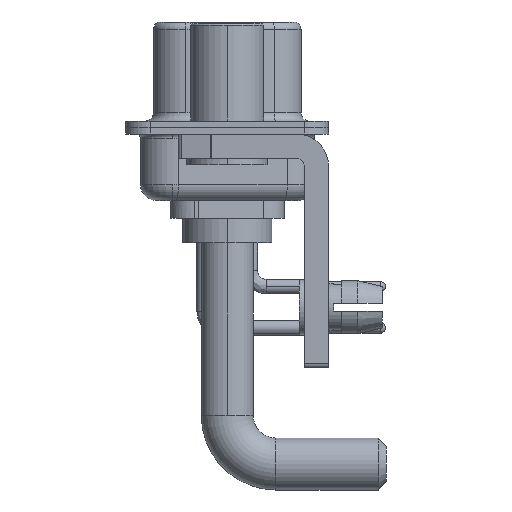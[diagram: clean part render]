
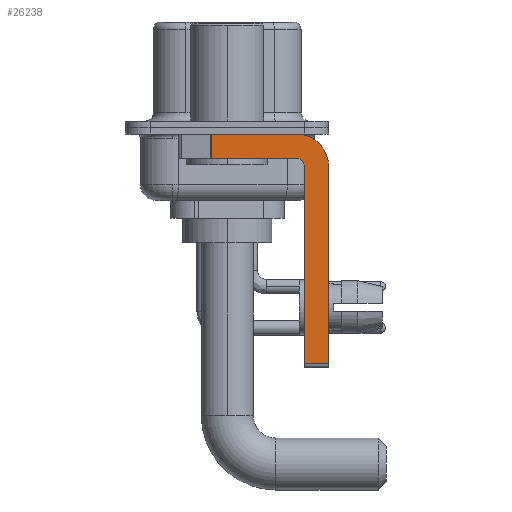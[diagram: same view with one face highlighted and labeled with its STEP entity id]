
A CAD part, left-side view. The second image highlights one B-rep face of the part: STEP entity #26238.
In plain terms, the highlighted planar face has unit normal (-1, 0, 0).
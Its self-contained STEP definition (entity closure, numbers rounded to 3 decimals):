
#71 = ORIENTED_EDGE ( 'NONE', *, *, #15314, .F. ) ;
#150 = CARTESIAN_POINT ( 'NONE',  ( -2.9, -4.25, -2.4 ) ) ;
#545 = CARTESIAN_POINT ( 'NONE',  ( -2.9, -4.25, -14.55 ) ) ;
#1232 = DIRECTION ( 'NONE',  ( -1., 0., 0. ) ) ;
#1467 = ORIENTED_EDGE ( 'NONE', *, *, #22378, .F. ) ;
#1584 = CARTESIAN_POINT ( 'NONE',  ( -2.9, -4.75, -2.4 ) ) ;
#1608 = VECTOR ( 'NONE', #7504, 1000. ) ;
#1879 = DIRECTION ( 'NONE',  ( 1., 0., 0. ) ) ;
#2025 = DIRECTION ( 'NONE',  ( 0., 0., -1. ) ) ;
#2563 = ORIENTED_EDGE ( 'NONE', *, *, #26449, .T. ) ;
#2705 = EDGE_LOOP ( 'NONE', ( #11683, #2563, #71, #1467, #7430, #20821, #26855, #7572 ) ) ;
#4264 = VECTOR ( 'NONE', #14315, 1000. ) ;
#5540 = CARTESIAN_POINT ( 'NONE',  ( -2.9, -6.25, -2.4 ) ) ;
#6569 = DIRECTION ( 'NONE',  ( 0., -1., 0. ) ) ;
#6678 = CIRCLE ( 'NONE', #23451, 2. ) ;
#7073 = LINE ( 'NONE', #20624, #1608 ) ;
#7117 = DIRECTION ( 'NONE',  ( 0., -1., 0. ) ) ;
#7430 = ORIENTED_EDGE ( 'NONE', *, *, #21015, .F. ) ;
#7504 = DIRECTION ( 'NONE',  ( 0., 0., 1. ) ) ;
#7505 = EDGE_CURVE ( 'NONE', #22199, #14180, #24375, .T. ) ;
#7572 = ORIENTED_EDGE ( 'NONE', *, *, #18465, .F. ) ;
#7615 = AXIS2_PLACEMENT_3D ( 'NONE', #12761, #1232, #8510 ) ;
#8292 = VERTEX_POINT ( 'NONE', #28421 ) ;
#8510 = DIRECTION ( 'NONE',  ( 0., 0., 1. ) ) ;
#8869 = CARTESIAN_POINT ( 'NONE',  ( -2.9, 0.978, -1.9 ) ) ;
#9920 = LINE ( 'NONE', #5540, #4264 ) ;
#10134 = VERTEX_POINT ( 'NONE', #26465 ) ;
#11087 = CARTESIAN_POINT ( 'NONE',  ( -2.9, 3., -0.4 ) ) ;
#11683 = ORIENTED_EDGE ( 'NONE', *, *, #7505, .F. ) ;
#12678 = CARTESIAN_POINT ( 'NONE',  ( -2.9, 0.978, -1.9 ) ) ;
#12738 = CARTESIAN_POINT ( 'NONE',  ( -2.9, -4.25, -1.9 ) ) ;
#12761 = CARTESIAN_POINT ( 'NONE',  ( -2.9, -4.25, -2.4 ) ) ;
#12811 = VERTEX_POINT ( 'NONE', #12738 ) ;
#13073 = EDGE_CURVE ( 'NONE', #8292, #20389, #9920, .T. ) ;
#13638 = VERTEX_POINT ( 'NONE', #1584 ) ;
#13811 = VECTOR ( 'NONE', #7117, 1000. ) ;
#14180 = VERTEX_POINT ( 'NONE', #19764 ) ;
#14315 = DIRECTION ( 'NONE',  ( 0., 0., -1. ) ) ;
#14385 = LINE ( 'NONE', #18903, #27163 ) ;
#15314 = EDGE_CURVE ( 'NONE', #12811, #18413, #14385, .T. ) ;
#15554 = CARTESIAN_POINT ( 'NONE',  ( -2.9, 0.978, -0.4 ) ) ;
#15763 = FACE_OUTER_BOUND ( 'NONE', #2705, .T. ) ;
#16015 = CARTESIAN_POINT ( 'NONE',  ( -2.9, -6.25, -14.55 ) ) ;
#18363 = CARTESIAN_POINT ( 'NONE',  ( -2.9, -4.25, -2.4 ) ) ;
#18413 = VERTEX_POINT ( 'NONE', #8869 ) ;
#18465 = EDGE_CURVE ( 'NONE', #14180, #8292, #6678, .T. ) ;
#18903 = CARTESIAN_POINT ( 'NONE',  ( -2.9, -4.25, -1.9 ) ) ;
#19764 = CARTESIAN_POINT ( 'NONE',  ( -2.9, -4.25, -0.4 ) ) ;
#19824 = VECTOR ( 'NONE', #2025, 1000. ) ;
#20389 = VERTEX_POINT ( 'NONE', #16015 ) ;
#20624 = CARTESIAN_POINT ( 'NONE',  ( -2.9, -4.75, -14.8 ) ) ;
#20754 = AXIS2_PLACEMENT_3D ( 'NONE', #150, #1879, #22744 ) ;
#20795 = DIRECTION ( 'NONE',  ( 0., 1., 0. ) ) ;
#20821 = ORIENTED_EDGE ( 'NONE', *, *, #26730, .T. ) ;
#20839 = LINE ( 'NONE', #12678, #19824 ) ;
#21015 = EDGE_CURVE ( 'NONE', #10134, #13638, #7073, .T. ) ;
#22199 = VERTEX_POINT ( 'NONE', #15554 ) ;
#22378 = EDGE_CURVE ( 'NONE', #13638, #12811, #24372, .T. ) ;
#22744 = DIRECTION ( 'NONE',  ( 0., 0., -1. ) ) ;
#23451 = AXIS2_PLACEMENT_3D ( 'NONE', #18363, #25754, #27278 ) ;
#24372 = CIRCLE ( 'NONE', #7615, 0.5 ) ;
#24375 = LINE ( 'NONE', #11087, #26717 ) ;
#25754 = DIRECTION ( 'NONE',  ( 1., 0., 0. ) ) ;
#26238 = ADVANCED_FACE ( 'NONE', ( #15763 ), #27306, .F. ) ;
#26449 = EDGE_CURVE ( 'NONE', #22199, #18413, #20839, .T. ) ;
#26465 = CARTESIAN_POINT ( 'NONE',  ( -2.9, -4.75, -14.55 ) ) ;
#26717 = VECTOR ( 'NONE', #6569, 1000. ) ;
#26730 = EDGE_CURVE ( 'NONE', #10134, #20389, #27111, .T. ) ;
#26855 = ORIENTED_EDGE ( 'NONE', *, *, #13073, .F. ) ;
#27111 = LINE ( 'NONE', #545, #13811 ) ;
#27163 = VECTOR ( 'NONE', #20795, 1000. ) ;
#27278 = DIRECTION ( 'NONE',  ( 0., 0., -1. ) ) ;
#27306 = PLANE ( 'NONE',  #20754 ) ;
#28421 = CARTESIAN_POINT ( 'NONE',  ( -2.9, -6.25, -2.4 ) ) ;
